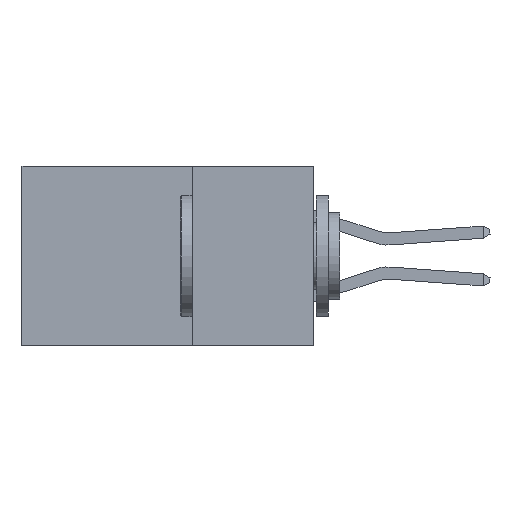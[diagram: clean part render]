
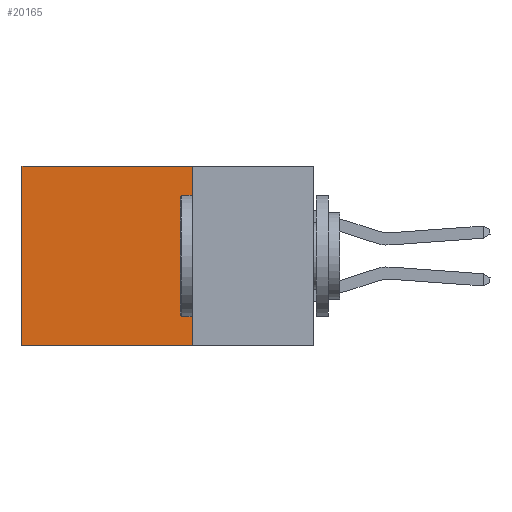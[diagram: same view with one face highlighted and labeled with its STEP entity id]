
A CAD part, left-side view. The second image highlights one B-rep face of the part: STEP entity #20165.
In plain terms, the highlighted planar face has unit normal (-1, 0, 0).
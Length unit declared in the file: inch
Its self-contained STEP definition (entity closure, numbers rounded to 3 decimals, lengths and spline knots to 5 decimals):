
#220 = EDGE_CURVE ( 'NONE', #3312, #28859, #4780, .T. ) ;
#1281 = LINE ( 'NONE', #5754, #8865 ) ;
#3312 = VERTEX_POINT ( 'NONE', #28574 ) ;
#3505 = ORIENTED_EDGE ( 'NONE', *, *, #6775, .F. ) ;
#3821 = DIRECTION ( 'NONE',  ( 0., 0., -1. ) ) ;
#4460 = VERTEX_POINT ( 'NONE', #19903 ) ;
#4681 = CARTESIAN_POINT ( 'NONE',  ( 0.2875, 0.25, -0.37 ) ) ;
#4780 = LINE ( 'NONE', #15202, #28903 ) ;
#5524 = VECTOR ( 'NONE', #33383, 39.37008 ) ;
#5754 = CARTESIAN_POINT ( 'NONE',  ( 0.2875, 0.25, 0. ) ) ;
#6097 = CARTESIAN_POINT ( 'NONE',  ( 0.2875, 0.25, -0.37 ) ) ;
#6604 = ORIENTED_EDGE ( 'NONE', *, *, #13448, .F. ) ;
#6775 = EDGE_CURVE ( 'NONE', #28729, #28859, #7809, .T. ) ;
#7809 = LINE ( 'NONE', #4681, #5524 ) ;
#8510 = FACE_OUTER_BOUND ( 'NONE', #35052, .T. ) ;
#8865 = VECTOR ( 'NONE', #19752, 39.37008 ) ;
#10258 = DIRECTION ( 'NONE',  ( 0., 0., -1. ) ) ;
#10621 = DIRECTION ( 'NONE',  ( 1., 0., 0. ) ) ;
#11314 = CARTESIAN_POINT ( 'NONE',  ( 0.2875, 0.25, 0. ) ) ;
#13448 = EDGE_CURVE ( 'NONE', #4460, #28729, #13782, .T. ) ;
#13782 = LINE ( 'NONE', #11314, #27128 ) ;
#14274 = ORIENTED_EDGE ( 'NONE', *, *, #220, .T. ) ;
#15202 = CARTESIAN_POINT ( 'NONE',  ( 0.2875, 0.6, 0. ) ) ;
#16901 = PLANE ( 'NONE',  #34172 ) ;
#19752 = DIRECTION ( 'NONE',  ( 0., 1., 0. ) ) ;
#19903 = CARTESIAN_POINT ( 'NONE',  ( 0.2875, 0.25, 0. ) ) ;
#20165 = ADVANCED_FACE ( 'NONE', ( #8510 ), #16901, .F. ) ;
#27128 = VECTOR ( 'NONE', #34935, 39.37008 ) ;
#28574 = CARTESIAN_POINT ( 'NONE',  ( 0.2875, 0.6, 0. ) ) ;
#28729 = VERTEX_POINT ( 'NONE', #6097 ) ;
#28859 = VERTEX_POINT ( 'NONE', #29939 ) ;
#28903 = VECTOR ( 'NONE', #3821, 39.37008 ) ;
#29572 = CARTESIAN_POINT ( 'NONE',  ( 0.2875, 0.25, 0. ) ) ;
#29939 = CARTESIAN_POINT ( 'NONE',  ( 0.2875, 0.6, -0.37 ) ) ;
#32357 = EDGE_CURVE ( 'NONE', #4460, #3312, #1281, .T. ) ;
#33383 = DIRECTION ( 'NONE',  ( 0., 1., 0. ) ) ;
#33728 = ORIENTED_EDGE ( 'NONE', *, *, #32357, .T. ) ;
#34172 = AXIS2_PLACEMENT_3D ( 'NONE', #29572, #10621, #10258 ) ;
#34935 = DIRECTION ( 'NONE',  ( 0., 0., -1. ) ) ;
#35052 = EDGE_LOOP ( 'NONE', ( #14274, #3505, #6604, #33728 ) ) ;
